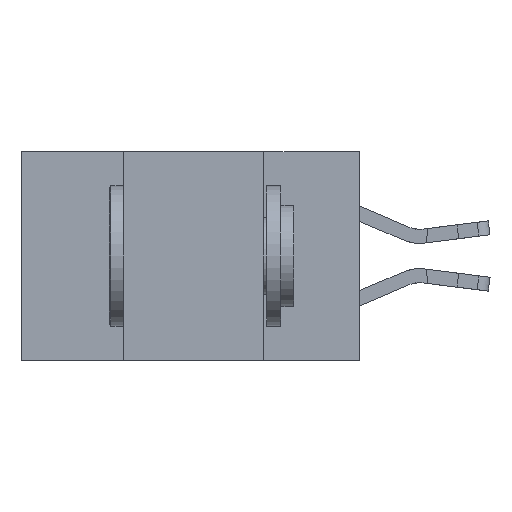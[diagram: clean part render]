
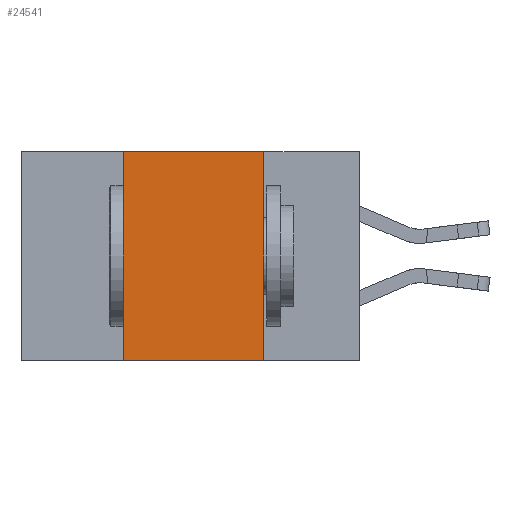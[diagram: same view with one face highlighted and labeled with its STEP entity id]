
A CAD part, left-side view. The second image highlights one B-rep face of the part: STEP entity #24541.
In plain terms, the highlighted planar face has unit normal (-1, 0, 0).
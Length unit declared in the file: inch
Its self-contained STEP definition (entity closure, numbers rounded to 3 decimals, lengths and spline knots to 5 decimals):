
#686 = VECTOR ( 'NONE', #6267, 39.37008 ) ;
#1673 = CARTESIAN_POINT ( 'NONE',  ( 0., 0.42, 0. ) ) ;
#1989 = ORIENTED_EDGE ( 'NONE', *, *, #2756, .F. ) ;
#2756 = EDGE_CURVE ( 'NONE', #10988, #16960, #23412, .T. ) ;
#3316 = EDGE_CURVE ( 'NONE', #16960, #5879, #8772, .T. ) ;
#4212 = CARTESIAN_POINT ( 'NONE',  ( 0., 0.6, -0.37 ) ) ;
#4940 = CARTESIAN_POINT ( 'NONE',  ( 0., 0.42, -0.37 ) ) ;
#5657 = ORIENTED_EDGE ( 'NONE', *, *, #3316, .F. ) ;
#5879 = VERTEX_POINT ( 'NONE', #20485 ) ;
#6267 = DIRECTION ( 'NONE',  ( 0., -1., 0. ) ) ;
#6703 = CARTESIAN_POINT ( 'NONE',  ( 0., 0.6, 0. ) ) ;
#7049 = FACE_OUTER_BOUND ( 'NONE', #10612, .T. ) ;
#7997 = DIRECTION ( 'NONE',  ( 0., 0., 1. ) ) ;
#8080 = LINE ( 'NONE', #8418, #10610 ) ;
#8418 = CARTESIAN_POINT ( 'NONE',  ( 0., 0.17, 0. ) ) ;
#8612 = EDGE_CURVE ( 'NONE', #5879, #14358, #8080, .T. ) ;
#8772 = LINE ( 'NONE', #24400, #24016 ) ;
#9777 = EDGE_CURVE ( 'NONE', #10988, #14358, #16900, .T. ) ;
#10444 = DIRECTION ( 'NONE',  ( 0., 0., -1. ) ) ;
#10610 = VECTOR ( 'NONE', #10444, 39.37008 ) ;
#10612 = EDGE_LOOP ( 'NONE', ( #13472, #5657, #1989, #16165 ) ) ;
#10950 = PLANE ( 'NONE',  #17173 ) ;
#10988 = VERTEX_POINT ( 'NONE', #4940 ) ;
#11576 = CARTESIAN_POINT ( 'NONE',  ( 0., 0.42, 0. ) ) ;
#12298 = DIRECTION ( 'NONE',  ( 0., -1., 0. ) ) ;
#13472 = ORIENTED_EDGE ( 'NONE', *, *, #8612, .F. ) ;
#14358 = VERTEX_POINT ( 'NONE', #18345 ) ;
#16165 = ORIENTED_EDGE ( 'NONE', *, *, #9777, .T. ) ;
#16900 = LINE ( 'NONE', #4212, #686 ) ;
#16960 = VERTEX_POINT ( 'NONE', #11576 ) ;
#17051 = VECTOR ( 'NONE', #7997, 39.37008 ) ;
#17173 = AXIS2_PLACEMENT_3D ( 'NONE', #6703, #19143, #19316 ) ;
#18345 = CARTESIAN_POINT ( 'NONE',  ( 0., 0.17, -0.37 ) ) ;
#19143 = DIRECTION ( 'NONE',  ( 1., 0., 0. ) ) ;
#19316 = DIRECTION ( 'NONE',  ( 0., 0., -1. ) ) ;
#20485 = CARTESIAN_POINT ( 'NONE',  ( 0., 0.17, 0. ) ) ;
#23412 = LINE ( 'NONE', #1673, #17051 ) ;
#24016 = VECTOR ( 'NONE', #12298, 39.37008 ) ;
#24400 = CARTESIAN_POINT ( 'NONE',  ( 0., 0.6, 0. ) ) ;
#24541 = ADVANCED_FACE ( 'NONE', ( #7049 ), #10950, .F. ) ;
